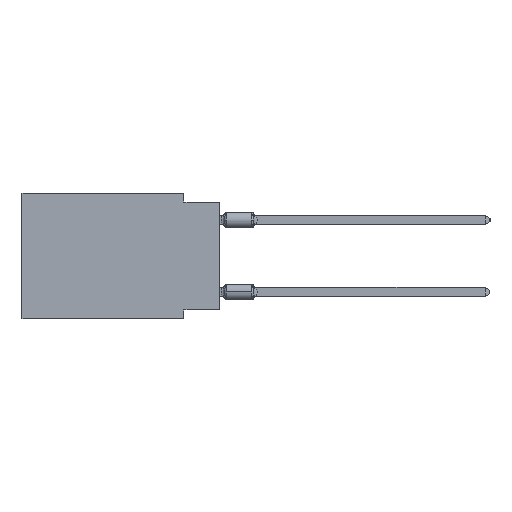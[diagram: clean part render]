
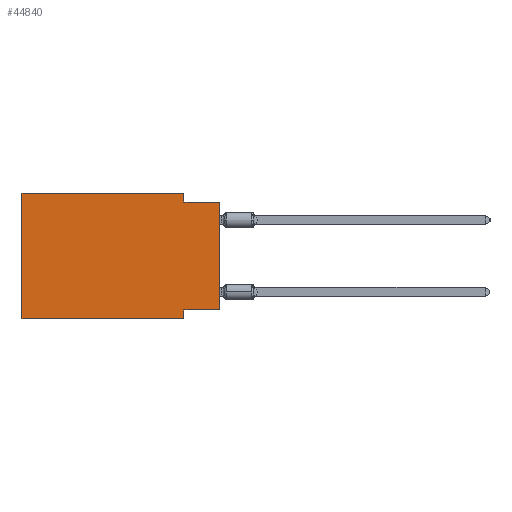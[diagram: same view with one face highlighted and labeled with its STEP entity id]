
A CAD part, left-side view. The second image highlights one B-rep face of the part: STEP entity #44840.
In plain terms, the highlighted planar face has unit normal (-1, 0, 0).
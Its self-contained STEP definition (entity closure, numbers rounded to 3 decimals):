
#36 = DIRECTION ( 'NONE',  ( 0., 0., -1. ) ) ;
#666 = ORIENTED_EDGE ( 'NONE', *, *, #46762, .F. ) ;
#985 = LINE ( 'NONE', #40853, #46183 ) ;
#1368 = EDGE_CURVE ( 'NONE', #35175, #39197, #31807, .T. ) ;
#1561 = VECTOR ( 'NONE', #33095, 1000. ) ;
#1782 = VERTEX_POINT ( 'NONE', #7708 ) ;
#2611 = CARTESIAN_POINT ( 'NONE',  ( 0., 13.97, 0. ) ) ;
#2950 = CARTESIAN_POINT ( 'NONE',  ( 0., 0., -8.255 ) ) ;
#3366 = VECTOR ( 'NONE', #17429, 1000. ) ;
#4127 = LINE ( 'NONE', #7963, #19385 ) ;
#4936 = CARTESIAN_POINT ( 'NONE',  ( 0., 2.54, -0.635 ) ) ;
#5804 = VERTEX_POINT ( 'NONE', #38722 ) ;
#5866 = ORIENTED_EDGE ( 'NONE', *, *, #38922, .F. ) ;
#6276 = LINE ( 'NONE', #34880, #44973 ) ;
#6880 = CARTESIAN_POINT ( 'NONE',  ( 0., 2.54, -8.255 ) ) ;
#7237 = CARTESIAN_POINT ( 'NONE',  ( 0., 2.54, -8.89 ) ) ;
#7708 = CARTESIAN_POINT ( 'NONE',  ( 0., 2.54, 0. ) ) ;
#7963 = CARTESIAN_POINT ( 'NONE',  ( 0., 0., -8.255 ) ) ;
#9771 = EDGE_LOOP ( 'NONE', ( #40352, #42182, #12941, #666, #5866, #39403, #45891, #21597 ) ) ;
#12036 = DIRECTION ( 'NONE',  ( 0., 0., 1. ) ) ;
#12941 = ORIENTED_EDGE ( 'NONE', *, *, #27314, .F. ) ;
#13469 = VERTEX_POINT ( 'NONE', #6880 ) ;
#13555 = DIRECTION ( 'NONE',  ( 0., -1., 0. ) ) ;
#13813 = LINE ( 'NONE', #42890, #3366 ) ;
#14602 = CARTESIAN_POINT ( 'NONE',  ( 0., 2.54, 0. ) ) ;
#14839 = LINE ( 'NONE', #14602, #1561 ) ;
#15723 = EDGE_CURVE ( 'NONE', #43247, #5804, #41655, .T. ) ;
#17429 = DIRECTION ( 'NONE',  ( 0., 0., 1. ) ) ;
#17987 = AXIS2_PLACEMENT_3D ( 'NONE', #21659, #43057, #32471 ) ;
#18580 = CARTESIAN_POINT ( 'NONE',  ( 0., 13.97, -8.89 ) ) ;
#18787 = EDGE_CURVE ( 'NONE', #13469, #5804, #25490, .T. ) ;
#19385 = VECTOR ( 'NONE', #22141, 1000. ) ;
#20929 = DIRECTION ( 'NONE',  ( 0., -1., 0. ) ) ;
#21350 = VERTEX_POINT ( 'NONE', #2950 ) ;
#21597 = ORIENTED_EDGE ( 'NONE', *, *, #37200, .F. ) ;
#21659 = CARTESIAN_POINT ( 'NONE',  ( 0., 13.97, 0. ) ) ;
#21901 = PLANE ( 'NONE',  #17987 ) ;
#22141 = DIRECTION ( 'NONE',  ( 0., 1., 0. ) ) ;
#24794 = FACE_OUTER_BOUND ( 'NONE', #9771, .T. ) ;
#25490 = LINE ( 'NONE', #7237, #34698 ) ;
#26772 = CARTESIAN_POINT ( 'NONE',  ( 0., 13.97, -8.89 ) ) ;
#27314 = EDGE_CURVE ( 'NONE', #1782, #35175, #14839, .T. ) ;
#27322 = VECTOR ( 'NONE', #13555, 1000. ) ;
#29949 = EDGE_CURVE ( 'NONE', #21350, #39197, #985, .T. ) ;
#31807 = LINE ( 'NONE', #46467, #27322 ) ;
#32194 = VERTEX_POINT ( 'NONE', #2611 ) ;
#32471 = DIRECTION ( 'NONE',  ( 0., 0., -1. ) ) ;
#33095 = DIRECTION ( 'NONE',  ( 0., 0., -1. ) ) ;
#33515 = VECTOR ( 'NONE', #44325, 1000. ) ;
#34698 = VECTOR ( 'NONE', #36, 1000. ) ;
#34880 = CARTESIAN_POINT ( 'NONE',  ( 0., 13.97, 0. ) ) ;
#35175 = VERTEX_POINT ( 'NONE', #4936 ) ;
#37200 = EDGE_CURVE ( 'NONE', #21350, #13469, #4127, .T. ) ;
#37807 = CARTESIAN_POINT ( 'NONE',  ( 0., 0., -0.635 ) ) ;
#38722 = CARTESIAN_POINT ( 'NONE',  ( 0., 2.54, -8.89 ) ) ;
#38922 = EDGE_CURVE ( 'NONE', #43247, #32194, #13813, .T. ) ;
#39197 = VERTEX_POINT ( 'NONE', #37807 ) ;
#39403 = ORIENTED_EDGE ( 'NONE', *, *, #15723, .T. ) ;
#40352 = ORIENTED_EDGE ( 'NONE', *, *, #29949, .T. ) ;
#40853 = CARTESIAN_POINT ( 'NONE',  ( 0., 0., 0. ) ) ;
#41655 = LINE ( 'NONE', #26772, #33515 ) ;
#42182 = ORIENTED_EDGE ( 'NONE', *, *, #1368, .F. ) ;
#42890 = CARTESIAN_POINT ( 'NONE',  ( 0., 13.97, 0. ) ) ;
#43057 = DIRECTION ( 'NONE',  ( 1., 0., 0. ) ) ;
#43247 = VERTEX_POINT ( 'NONE', #18580 ) ;
#44325 = DIRECTION ( 'NONE',  ( 0., -1., 0. ) ) ;
#44840 = ADVANCED_FACE ( 'NONE', ( #24794 ), #21901, .F. ) ;
#44973 = VECTOR ( 'NONE', #20929, 1000. ) ;
#45891 = ORIENTED_EDGE ( 'NONE', *, *, #18787, .F. ) ;
#46183 = VECTOR ( 'NONE', #12036, 1000. ) ;
#46467 = CARTESIAN_POINT ( 'NONE',  ( 0., 0., -0.635 ) ) ;
#46762 = EDGE_CURVE ( 'NONE', #32194, #1782, #6276, .T. ) ;
